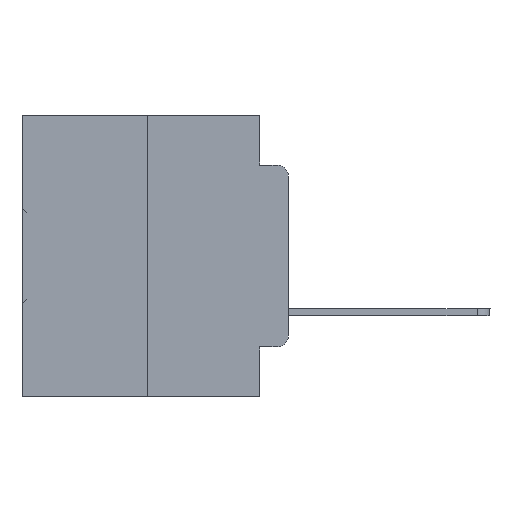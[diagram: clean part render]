
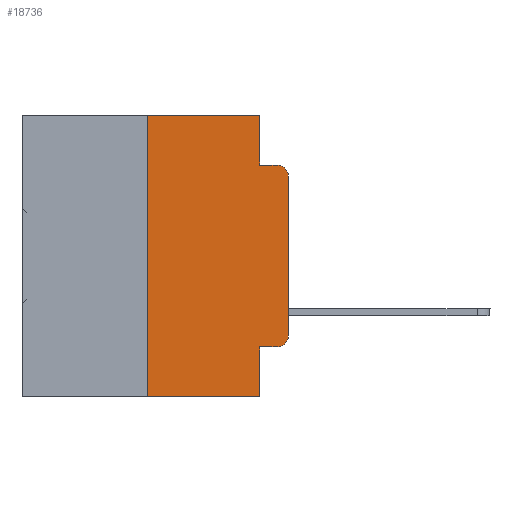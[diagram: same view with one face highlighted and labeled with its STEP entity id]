
A CAD part, left-side view. The second image highlights one B-rep face of the part: STEP entity #18736.
In plain terms, the highlighted planar face has unit normal (-1, 0, 0).
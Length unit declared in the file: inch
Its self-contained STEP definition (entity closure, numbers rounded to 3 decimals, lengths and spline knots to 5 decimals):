
#286 = CIRCLE ( 'NONE', #23122, 0.02 ) ;
#328 = EDGE_CURVE ( 'NONE', #19586, #9381, #824, .T. ) ;
#574 = CARTESIAN_POINT ( 'NONE',  ( 0., 0., -0.3915 ) ) ;
#808 = VECTOR ( 'NONE', #21150, 39.37008 ) ;
#824 = LINE ( 'NONE', #18576, #808 ) ;
#857 = DIRECTION ( 'NONE',  ( 0., 0., -1. ) ) ;
#1103 = EDGE_CURVE ( 'NONE', #32257, #6223, #21851, .T. ) ;
#1258 = DIRECTION ( 'NONE',  ( 1., 0., 0. ) ) ;
#1587 = EDGE_CURVE ( 'NONE', #23193, #3893, #22478, .T. ) ;
#1805 = EDGE_CURVE ( 'NONE', #9381, #16926, #11313, .T. ) ;
#3367 = CARTESIAN_POINT ( 'NONE',  ( 0., 0.25, -0.5 ) ) ;
#3519 = ORIENTED_EDGE ( 'NONE', *, *, #1103, .T. ) ;
#3735 = CARTESIAN_POINT ( 'NONE',  ( 0., 0.051, -0.4115 ) ) ;
#3893 = VERTEX_POINT ( 'NONE', #15528 ) ;
#3956 = DIRECTION ( 'NONE',  ( 0., 0., -1. ) ) ;
#5027 = CARTESIAN_POINT ( 'NONE',  ( 0., 0.473, -0.5 ) ) ;
#5198 = CARTESIAN_POINT ( 'NONE',  ( 0., 0., -0.1085 ) ) ;
#6223 = VERTEX_POINT ( 'NONE', #5198 ) ;
#6928 = EDGE_CURVE ( 'NONE', #20463, #33106, #26109, .T. ) ;
#7488 = CARTESIAN_POINT ( 'NONE',  ( 0., 0.051, -0.0885 ) ) ;
#7518 = LINE ( 'NONE', #17926, #25907 ) ;
#7654 = DIRECTION ( 'NONE',  ( 0., -1., 0. ) ) ;
#8084 = DIRECTION ( 'NONE',  ( 0., -1., 0. ) ) ;
#8430 = CIRCLE ( 'NONE', #25350, 0.02 ) ;
#8841 = DIRECTION ( 'NONE',  ( 0., 0., 1. ) ) ;
#9153 = CARTESIAN_POINT ( 'NONE',  ( 0., 0.02, -0.1085 ) ) ;
#9175 = AXIS2_PLACEMENT_3D ( 'NONE', #27398, #1258, #3956 ) ;
#9381 = VERTEX_POINT ( 'NONE', #24967 ) ;
#10716 = CARTESIAN_POINT ( 'NONE',  ( 0., 0.051, 0. ) ) ;
#10764 = CARTESIAN_POINT ( 'NONE',  ( 0., 0.051, -0.5 ) ) ;
#11313 = LINE ( 'NONE', #29295, #24359 ) ;
#11378 = ORIENTED_EDGE ( 'NONE', *, *, #1805, .F. ) ;
#11437 = CARTESIAN_POINT ( 'NONE',  ( 0., 0.051, -0.0885 ) ) ;
#11731 = VECTOR ( 'NONE', #25555, 39.37008 ) ;
#12292 = ORIENTED_EDGE ( 'NONE', *, *, #21689, .F. ) ;
#12742 = EDGE_CURVE ( 'NONE', #19586, #28380, #23663, .T. ) ;
#14778 = ORIENTED_EDGE ( 'NONE', *, *, #27574, .F. ) ;
#14826 = DIRECTION ( 'NONE',  ( 0., 0., -1. ) ) ;
#15497 = DIRECTION ( 'NONE',  ( -1., 0., 0. ) ) ;
#15528 = CARTESIAN_POINT ( 'NONE',  ( 0., 0.02, -0.4115 ) ) ;
#15669 = ORIENTED_EDGE ( 'NONE', *, *, #328, .F. ) ;
#16473 = CARTESIAN_POINT ( 'NONE',  ( 0., 0.051, 0. ) ) ;
#16678 = DIRECTION ( 'NONE',  ( -1., 0., 0. ) ) ;
#16926 = VERTEX_POINT ( 'NONE', #16473 ) ;
#16946 = FACE_OUTER_BOUND ( 'NONE', #19212, .T. ) ;
#17926 = CARTESIAN_POINT ( 'NONE',  ( 0., 0.051, 0. ) ) ;
#18576 = CARTESIAN_POINT ( 'NONE',  ( 0., 0.25, 0. ) ) ;
#18736 = ADVANCED_FACE ( 'NONE', ( #16946 ), #24665, .F. ) ;
#18950 = LINE ( 'NONE', #10716, #23413 ) ;
#19213 = ORIENTED_EDGE ( 'NONE', *, *, #6928, .F. ) ;
#19212 = EDGE_LOOP ( 'NONE', ( #3519, #30543, #19213, #12292, #11378, #15669, #22532, #14778, #27091, #22502 ) ) ;
#19586 = VERTEX_POINT ( 'NONE', #3367 ) ;
#19599 = DIRECTION ( 'NONE',  ( 0., 0., -1. ) ) ;
#19984 = VECTOR ( 'NONE', #22805, 39.37008 ) ;
#20342 = DIRECTION ( 'NONE',  ( 0., 0., -1. ) ) ;
#20463 = VERTEX_POINT ( 'NONE', #11437 ) ;
#20912 = VECTOR ( 'NONE', #8841, 39.37008 ) ;
#21150 = DIRECTION ( 'NONE',  ( 0., 0., 1. ) ) ;
#21383 = VECTOR ( 'NONE', #7654, 39.37008 ) ;
#21689 = EDGE_CURVE ( 'NONE', #16926, #20463, #7518, .T. ) ;
#21851 = LINE ( 'NONE', #32256, #20912 ) ;
#22409 = EDGE_CURVE ( 'NONE', #6223, #33106, #286, .T. ) ;
#22478 = LINE ( 'NONE', #32892, #19984 ) ;
#22502 = ORIENTED_EDGE ( 'NONE', *, *, #23280, .T. ) ;
#22532 = ORIENTED_EDGE ( 'NONE', *, *, #12742, .T. ) ;
#22805 = DIRECTION ( 'NONE',  ( 0., -1., 0. ) ) ;
#23122 = AXIS2_PLACEMENT_3D ( 'NONE', #9153, #16678, #19599 ) ;
#23193 = VERTEX_POINT ( 'NONE', #3735 ) ;
#23280 = EDGE_CURVE ( 'NONE', #3893, #32257, #8430, .T. ) ;
#23413 = VECTOR ( 'NONE', #857, 39.37008 ) ;
#23663 = LINE ( 'NONE', #5027, #11731 ) ;
#24359 = VECTOR ( 'NONE', #8084, 39.37008 ) ;
#24665 = PLANE ( 'NONE',  #9175 ) ;
#24967 = CARTESIAN_POINT ( 'NONE',  ( 0., 0.25, 0. ) ) ;
#25350 = AXIS2_PLACEMENT_3D ( 'NONE', #28518, #15497, #14826 ) ;
#25555 = DIRECTION ( 'NONE',  ( 0., -1., 0. ) ) ;
#25907 = VECTOR ( 'NONE', #20342, 39.37008 ) ;
#26109 = LINE ( 'NONE', #7488, #21383 ) ;
#27091 = ORIENTED_EDGE ( 'NONE', *, *, #1587, .T. ) ;
#27398 = CARTESIAN_POINT ( 'NONE',  ( 0., 0.473, 0. ) ) ;
#27574 = EDGE_CURVE ( 'NONE', #23193, #28380, #18950, .T. ) ;
#28380 = VERTEX_POINT ( 'NONE', #10764 ) ;
#28518 = CARTESIAN_POINT ( 'NONE',  ( 0., 0.02, -0.3915 ) ) ;
#29295 = CARTESIAN_POINT ( 'NONE',  ( 0., 0.473, 0. ) ) ;
#30089 = CARTESIAN_POINT ( 'NONE',  ( 0., 0.02, -0.0885 ) ) ;
#30543 = ORIENTED_EDGE ( 'NONE', *, *, #22409, .T. ) ;
#32256 = CARTESIAN_POINT ( 'NONE',  ( 0., 0., 0. ) ) ;
#32257 = VERTEX_POINT ( 'NONE', #574 ) ;
#32892 = CARTESIAN_POINT ( 'NONE',  ( 0., 0.051, -0.4115 ) ) ;
#33106 = VERTEX_POINT ( 'NONE', #30089 ) ;
